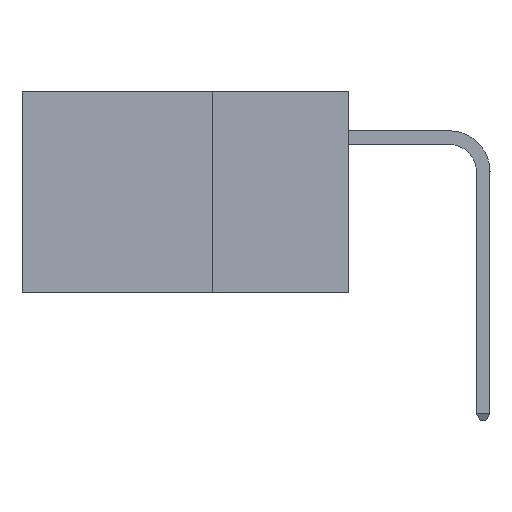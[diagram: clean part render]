
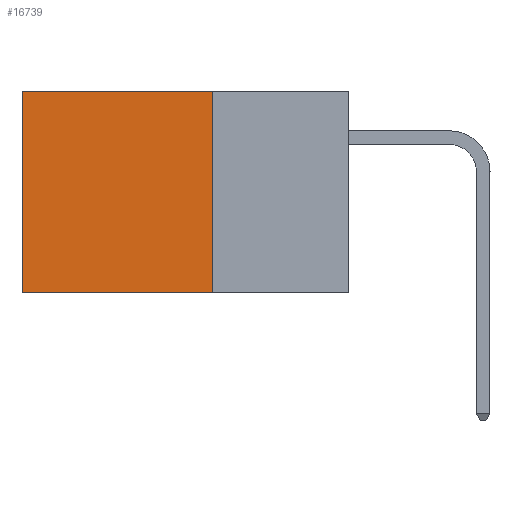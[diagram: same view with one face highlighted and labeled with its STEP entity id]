
A CAD part, left-side view. The second image highlights one B-rep face of the part: STEP entity #16739.
In plain terms, the highlighted planar face has unit normal (-1, 0, 0).
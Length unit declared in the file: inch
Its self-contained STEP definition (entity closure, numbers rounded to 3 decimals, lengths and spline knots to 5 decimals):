
#930 = VECTOR ( 'NONE', #17177, 39.37008 ) ;
#1293 = EDGE_CURVE ( 'NONE', #8428, #13438, #15591, .T. ) ;
#2317 = VERTEX_POINT ( 'NONE', #8096 ) ;
#2758 = EDGE_CURVE ( 'NONE', #15145, #2317, #16677, .T. ) ;
#2989 = LINE ( 'NONE', #14965, #17873 ) ;
#3338 = ORIENTED_EDGE ( 'NONE', *, *, #12182, .T. ) ;
#3539 = CARTESIAN_POINT ( 'NONE',  ( 0.2875, 0.25, 0. ) ) ;
#3743 = VECTOR ( 'NONE', #18121, 39.37008 ) ;
#4928 = CARTESIAN_POINT ( 'NONE',  ( 0.2875, 0.25, -0.37 ) ) ;
#5866 = ORIENTED_EDGE ( 'NONE', *, *, #2758, .F. ) ;
#7496 = EDGE_LOOP ( 'NONE', ( #12923, #19815, #5866, #3338 ) ) ;
#8096 = CARTESIAN_POINT ( 'NONE',  ( 0.2875, 0.25, -0.37 ) ) ;
#8307 = DIRECTION ( 'NONE',  ( 1., 0., 0. ) ) ;
#8428 = VERTEX_POINT ( 'NONE', #9079 ) ;
#9079 = CARTESIAN_POINT ( 'NONE',  ( 0.2875, 0.6, 0. ) ) ;
#9845 = PLANE ( 'NONE',  #11984 ) ;
#10013 = CARTESIAN_POINT ( 'NONE',  ( 0.2875, 0.25, 0. ) ) ;
#11984 = AXIS2_PLACEMENT_3D ( 'NONE', #3539, #8307, #18814 ) ;
#12182 = EDGE_CURVE ( 'NONE', #15145, #8428, #2989, .T. ) ;
#12734 = VECTOR ( 'NONE', #17475, 39.37008 ) ;
#12923 = ORIENTED_EDGE ( 'NONE', *, *, #1293, .T. ) ;
#13058 = EDGE_CURVE ( 'NONE', #2317, #13438, #13463, .T. ) ;
#13307 = FACE_OUTER_BOUND ( 'NONE', #7496, .T. ) ;
#13438 = VERTEX_POINT ( 'NONE', #13690 ) ;
#13463 = LINE ( 'NONE', #4928, #930 ) ;
#13690 = CARTESIAN_POINT ( 'NONE',  ( 0.2875, 0.6, -0.37 ) ) ;
#14965 = CARTESIAN_POINT ( 'NONE',  ( 0.2875, 0.25, 0. ) ) ;
#15145 = VERTEX_POINT ( 'NONE', #10013 ) ;
#15591 = LINE ( 'NONE', #17590, #3743 ) ;
#16677 = LINE ( 'NONE', #17368, #12734 ) ;
#16739 = ADVANCED_FACE ( 'NONE', ( #13307 ), #9845, .F. ) ;
#17177 = DIRECTION ( 'NONE',  ( 0., 1., 0. ) ) ;
#17368 = CARTESIAN_POINT ( 'NONE',  ( 0.2875, 0.25, 0. ) ) ;
#17475 = DIRECTION ( 'NONE',  ( 0., 0., -1. ) ) ;
#17590 = CARTESIAN_POINT ( 'NONE',  ( 0.2875, 0.6, 0. ) ) ;
#17873 = VECTOR ( 'NONE', #19369, 39.37008 ) ;
#18121 = DIRECTION ( 'NONE',  ( 0., 0., -1. ) ) ;
#18814 = DIRECTION ( 'NONE',  ( 0., 0., -1. ) ) ;
#19369 = DIRECTION ( 'NONE',  ( 0., 1., 0. ) ) ;
#19815 = ORIENTED_EDGE ( 'NONE', *, *, #13058, .F. ) ;
